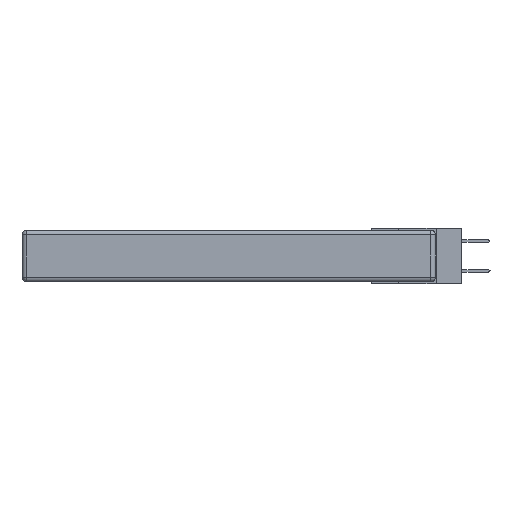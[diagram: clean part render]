
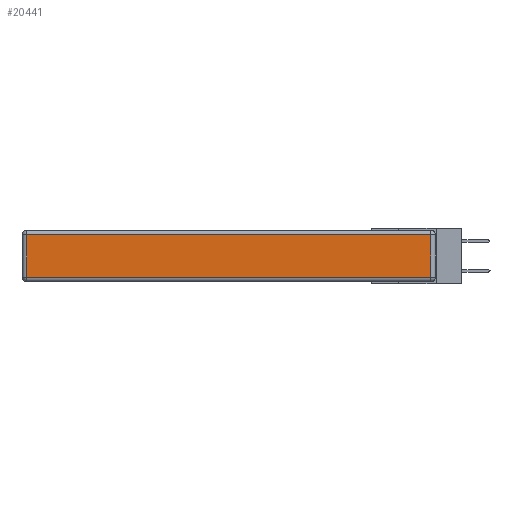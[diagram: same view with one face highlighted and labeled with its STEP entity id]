
A CAD part, left-side view. The second image highlights one B-rep face of the part: STEP entity #20441.
In plain terms, the highlighted planar face has unit normal (-1, 0, 0).
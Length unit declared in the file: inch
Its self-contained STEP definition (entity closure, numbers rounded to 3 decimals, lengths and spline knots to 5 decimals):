
#403 = VERTEX_POINT ( 'NONE', #15272 ) ;
#3509 = VECTOR ( 'NONE', #12035, 39.37008 ) ;
#4523 = DIRECTION ( 'NONE',  ( 0., 0., 1. ) ) ;
#6931 = AXIS2_PLACEMENT_3D ( 'NONE', #13424, #17607, #25681 ) ;
#7624 = DIRECTION ( 'NONE',  ( 0., 0., -1. ) ) ;
#8330 = EDGE_CURVE ( 'NONE', #403, #20485, #22054, .T. ) ;
#9923 = DIRECTION ( 'NONE',  ( 0., -1., 0. ) ) ;
#9936 = CARTESIAN_POINT ( 'NONE',  ( 0., 2.75, -0.03 ) ) ;
#10930 = EDGE_LOOP ( 'NONE', ( #18506, #21483, #13813, #24855 ) ) ;
#12035 = DIRECTION ( 'NONE',  ( 0., 1., 0. ) ) ;
#13232 = VECTOR ( 'NONE', #4523, 39.37008 ) ;
#13378 = VECTOR ( 'NONE', #7624, 39.37008 ) ;
#13424 = CARTESIAN_POINT ( 'NONE',  ( 0., 0., -0.343 ) ) ;
#13518 = CARTESIAN_POINT ( 'NONE',  ( 0., 0.03, -0.313 ) ) ;
#13813 = ORIENTED_EDGE ( 'NONE', *, *, #23533, .T. ) ;
#14200 = VERTEX_POINT ( 'NONE', #23833 ) ;
#14263 = FACE_OUTER_BOUND ( 'NONE', #10930, .T. ) ;
#15272 = CARTESIAN_POINT ( 'NONE',  ( 0., 2.72, -0.313 ) ) ;
#15334 = CARTESIAN_POINT ( 'NONE',  ( 0., 2.72, -0.343 ) ) ;
#16200 = LINE ( 'NONE', #15334, #13378 ) ;
#16543 = CARTESIAN_POINT ( 'NONE',  ( 0., 0.03, -0.343 ) ) ;
#16788 = VECTOR ( 'NONE', #9923, 39.37008 ) ;
#17607 = DIRECTION ( 'NONE',  ( -1., 0., 0. ) ) ;
#18506 = ORIENTED_EDGE ( 'NONE', *, *, #8330, .T. ) ;
#19125 = LINE ( 'NONE', #16543, #13232 ) ;
#19308 = EDGE_CURVE ( 'NONE', #19967, #403, #16200, .T. ) ;
#19967 = VERTEX_POINT ( 'NONE', #25464 ) ;
#20441 = ADVANCED_FACE ( 'NONE', ( #14263 ), #23610, .T. ) ;
#20485 = VERTEX_POINT ( 'NONE', #13518 ) ;
#21312 = EDGE_CURVE ( 'NONE', #20485, #14200, #19125, .T. ) ;
#21483 = ORIENTED_EDGE ( 'NONE', *, *, #21312, .T. ) ;
#22054 = LINE ( 'NONE', #23707, #16788 ) ;
#23533 = EDGE_CURVE ( 'NONE', #14200, #19967, #24174, .T. ) ;
#23610 = PLANE ( 'NONE',  #6931 ) ;
#23707 = CARTESIAN_POINT ( 'NONE',  ( 0., 0., -0.313 ) ) ;
#23833 = CARTESIAN_POINT ( 'NONE',  ( 0., 0.03, -0.03 ) ) ;
#24174 = LINE ( 'NONE', #9936, #3509 ) ;
#24855 = ORIENTED_EDGE ( 'NONE', *, *, #19308, .T. ) ;
#25464 = CARTESIAN_POINT ( 'NONE',  ( 0., 2.72, -0.03 ) ) ;
#25681 = DIRECTION ( 'NONE',  ( 0., 0., 1. ) ) ;
